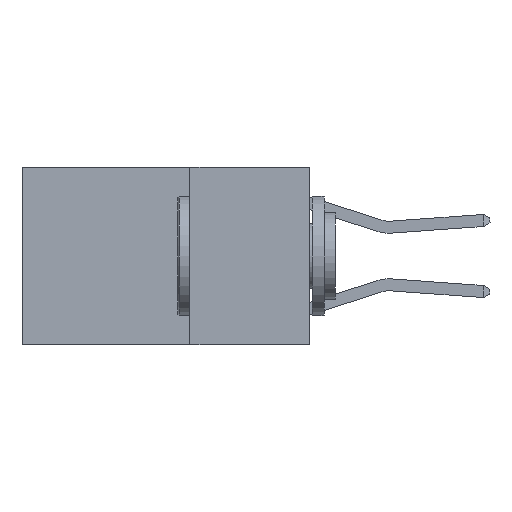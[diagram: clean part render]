
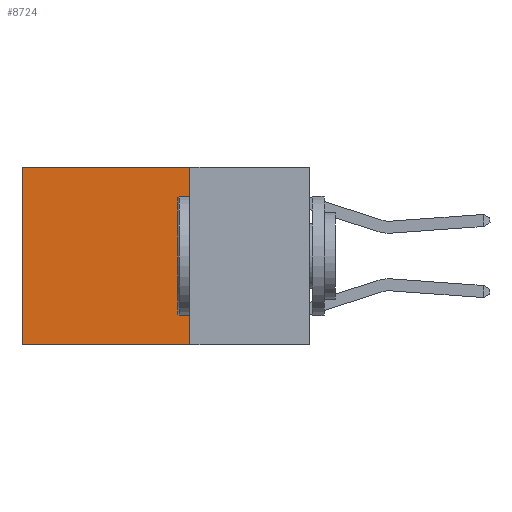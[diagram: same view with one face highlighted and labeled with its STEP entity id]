
A CAD part, left-side view. The second image highlights one B-rep face of the part: STEP entity #8724.
In plain terms, the highlighted planar face has unit normal (-1, 0, 0).
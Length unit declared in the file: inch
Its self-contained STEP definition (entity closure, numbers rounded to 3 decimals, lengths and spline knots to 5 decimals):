
#425 = VECTOR ( 'NONE', #5961, 39.37008 ) ;
#1619 = PLANE ( 'NONE',  #5731 ) ;
#1972 = LINE ( 'NONE', #21395, #21533 ) ;
#3303 = DIRECTION ( 'NONE',  ( 0., 1., 0. ) ) ;
#4016 = VECTOR ( 'NONE', #11790, 39.37008 ) ;
#5206 = FACE_OUTER_BOUND ( 'NONE', #19234, .T. ) ;
#5671 = LINE ( 'NONE', #21027, #425 ) ;
#5731 = AXIS2_PLACEMENT_3D ( 'NONE', #20652, #9380, #22494 ) ;
#5946 = CARTESIAN_POINT ( 'NONE',  ( 0.2625, 0.25, -0.37 ) ) ;
#5961 = DIRECTION ( 'NONE',  ( 0., 0., -1. ) ) ;
#5988 = CARTESIAN_POINT ( 'NONE',  ( 0.2625, 0.25, 0. ) ) ;
#6160 = CARTESIAN_POINT ( 'NONE',  ( 0.2625, 0.25, -0.37 ) ) ;
#8724 = ADVANCED_FACE ( 'NONE', ( #5206 ), #1619, .F. ) ;
#9037 = VECTOR ( 'NONE', #3303, 39.37008 ) ;
#9380 = DIRECTION ( 'NONE',  ( 1., 0., 0. ) ) ;
#9522 = CARTESIAN_POINT ( 'NONE',  ( 0.2625, 0.6, -0.37 ) ) ;
#10206 = VERTEX_POINT ( 'NONE', #5946 ) ;
#11790 = DIRECTION ( 'NONE',  ( 0., 1., 0. ) ) ;
#12365 = LINE ( 'NONE', #6160, #4016 ) ;
#13155 = EDGE_CURVE ( 'NONE', #21283, #21878, #22808, .T. ) ;
#14688 = CARTESIAN_POINT ( 'NONE',  ( 0.2625, 0.25, 0. ) ) ;
#14790 = EDGE_CURVE ( 'NONE', #21878, #23902, #5671, .T. ) ;
#16422 = EDGE_CURVE ( 'NONE', #21283, #10206, #1972, .T. ) ;
#17092 = ORIENTED_EDGE ( 'NONE', *, *, #16422, .F. ) ;
#19064 = EDGE_CURVE ( 'NONE', #10206, #23902, #12365, .T. ) ;
#19234 = EDGE_LOOP ( 'NONE', ( #21470, #19332, #17092, #19887 ) ) ;
#19332 = ORIENTED_EDGE ( 'NONE', *, *, #19064, .F. ) ;
#19887 = ORIENTED_EDGE ( 'NONE', *, *, #13155, .T. ) ;
#20652 = CARTESIAN_POINT ( 'NONE',  ( 0.2625, 0.25, 0. ) ) ;
#21027 = CARTESIAN_POINT ( 'NONE',  ( 0.2625, 0.6, 0. ) ) ;
#21283 = VERTEX_POINT ( 'NONE', #5988 ) ;
#21395 = CARTESIAN_POINT ( 'NONE',  ( 0.2625, 0.25, 0. ) ) ;
#21470 = ORIENTED_EDGE ( 'NONE', *, *, #14790, .T. ) ;
#21533 = VECTOR ( 'NONE', #23246, 39.37008 ) ;
#21878 = VERTEX_POINT ( 'NONE', #24343 ) ;
#22494 = DIRECTION ( 'NONE',  ( 0., 0., -1. ) ) ;
#22808 = LINE ( 'NONE', #14688, #9037 ) ;
#23246 = DIRECTION ( 'NONE',  ( 0., 0., -1. ) ) ;
#23902 = VERTEX_POINT ( 'NONE', #9522 ) ;
#24343 = CARTESIAN_POINT ( 'NONE',  ( 0.2625, 0.6, 0. ) ) ;
